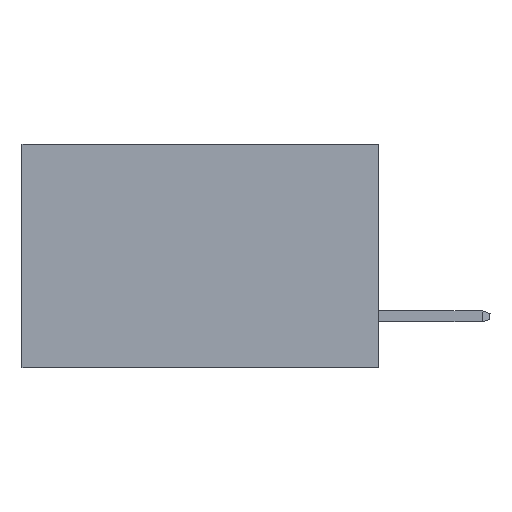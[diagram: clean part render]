
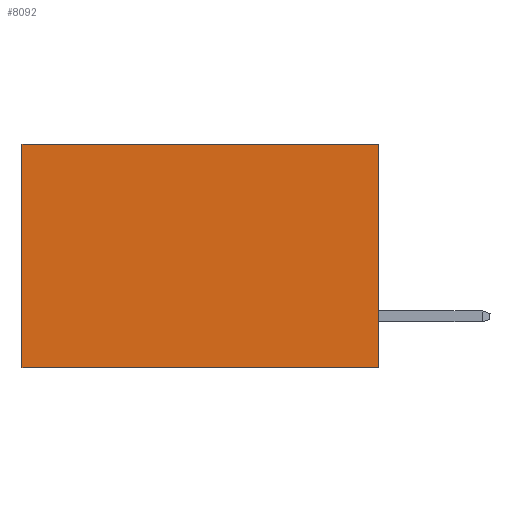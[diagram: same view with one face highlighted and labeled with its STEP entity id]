
A CAD part, left-side view. The second image highlights one B-rep face of the part: STEP entity #8092.
In plain terms, the highlighted planar face has unit normal (-1, 0, 0).
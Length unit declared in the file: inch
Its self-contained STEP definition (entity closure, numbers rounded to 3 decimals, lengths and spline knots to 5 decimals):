
#1150 = LINE ( 'NONE', #21720, #19304 ) ;
#2096 = EDGE_LOOP ( 'NONE', ( #17546, #8463, #13872, #18682 ) ) ;
#2157 = CARTESIAN_POINT ( 'NONE',  ( 0.277, 0., 0. ) ) ;
#2409 = VECTOR ( 'NONE', #19714, 39.37008 ) ;
#3504 = VECTOR ( 'NONE', #5365, 39.37008 ) ;
#3950 = CARTESIAN_POINT ( 'NONE',  ( 0.277, 0., 0. ) ) ;
#4539 = EDGE_CURVE ( 'NONE', #5703, #12003, #6709, .T. ) ;
#5365 = DIRECTION ( 'NONE',  ( 0., 0., -1. ) ) ;
#5703 = VERTEX_POINT ( 'NONE', #7825 ) ;
#5727 = EDGE_CURVE ( 'NONE', #14281, #12003, #17957, .T. ) ;
#5984 = VECTOR ( 'NONE', #20257, 39.37008 ) ;
#6700 = DIRECTION ( 'NONE',  ( 0., 0., -1. ) ) ;
#6709 = LINE ( 'NONE', #19737, #2409 ) ;
#7131 = FACE_OUTER_BOUND ( 'NONE', #2096, .T. ) ;
#7630 = CARTESIAN_POINT ( 'NONE',  ( 0.277, 0.59, -0.37 ) ) ;
#7825 = CARTESIAN_POINT ( 'NONE',  ( 0.277, 0., -0.37 ) ) ;
#8092 = ADVANCED_FACE ( 'NONE', ( #7131 ), #15710, .F. ) ;
#8463 = ORIENTED_EDGE ( 'NONE', *, *, #4539, .F. ) ;
#12003 = VERTEX_POINT ( 'NONE', #23061 ) ;
#12835 = DIRECTION ( 'NONE',  ( 0., 0., -1. ) ) ;
#13872 = ORIENTED_EDGE ( 'NONE', *, *, #14734, .F. ) ;
#14281 = VERTEX_POINT ( 'NONE', #18194 ) ;
#14734 = EDGE_CURVE ( 'NONE', #18945, #5703, #1150, .T. ) ;
#15710 = PLANE ( 'NONE',  #21905 ) ;
#16235 = EDGE_CURVE ( 'NONE', #18945, #14281, #19795, .T. ) ;
#17509 = DIRECTION ( 'NONE',  ( 1., 0., 0. ) ) ;
#17546 = ORIENTED_EDGE ( 'NONE', *, *, #5727, .T. ) ;
#17957 = LINE ( 'NONE', #7630, #3504 ) ;
#18194 = CARTESIAN_POINT ( 'NONE',  ( 0.277, 0.59, 0. ) ) ;
#18682 = ORIENTED_EDGE ( 'NONE', *, *, #16235, .T. ) ;
#18945 = VERTEX_POINT ( 'NONE', #3950 ) ;
#19304 = VECTOR ( 'NONE', #12835, 39.37008 ) ;
#19714 = DIRECTION ( 'NONE',  ( 0., 1., 0. ) ) ;
#19737 = CARTESIAN_POINT ( 'NONE',  ( 0.277, 0., -0.37 ) ) ;
#19795 = LINE ( 'NONE', #2157, #5984 ) ;
#20257 = DIRECTION ( 'NONE',  ( 0., 1., 0. ) ) ;
#21720 = CARTESIAN_POINT ( 'NONE',  ( 0.277, 0., -0.37 ) ) ;
#21905 = AXIS2_PLACEMENT_3D ( 'NONE', #22765, #17509, #6700 ) ;
#22765 = CARTESIAN_POINT ( 'NONE',  ( 0.277, 0., -0.37 ) ) ;
#23061 = CARTESIAN_POINT ( 'NONE',  ( 0.277, 0.59, -0.37 ) ) ;
